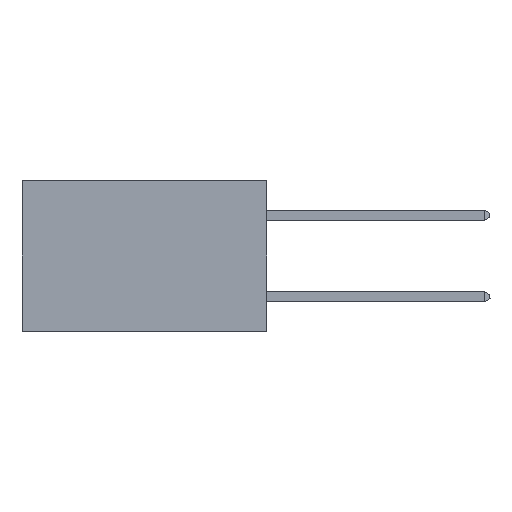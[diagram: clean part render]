
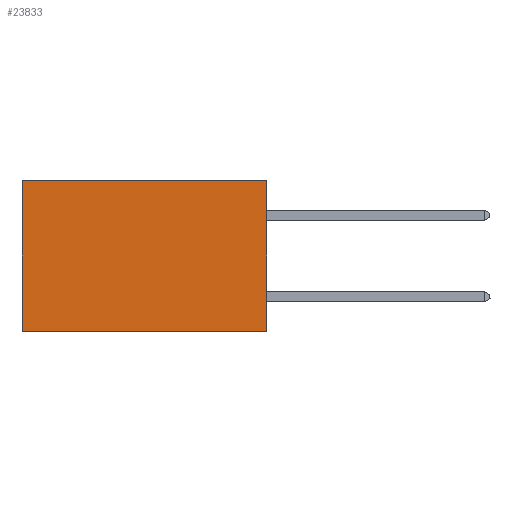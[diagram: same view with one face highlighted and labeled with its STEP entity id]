
A CAD part, left-side view. The second image highlights one B-rep face of the part: STEP entity #23833.
In plain terms, the highlighted planar face has unit normal (-1, 0, 0).
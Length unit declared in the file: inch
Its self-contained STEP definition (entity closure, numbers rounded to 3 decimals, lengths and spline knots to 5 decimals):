
#265 = VERTEX_POINT ( 'NONE', #5550 ) ;
#536 = EDGE_CURVE ( 'NONE', #12801, #21886, #4469, .T. ) ;
#2067 = DIRECTION ( 'NONE',  ( 0., 0., -1. ) ) ;
#2367 = LINE ( 'NONE', #5290, #14525 ) ;
#3176 = CARTESIAN_POINT ( 'NONE',  ( 0.2875, 0., -0.37 ) ) ;
#3340 = ORIENTED_EDGE ( 'NONE', *, *, #536, .T. ) ;
#3787 = LINE ( 'NONE', #24028, #14053 ) ;
#4469 = LINE ( 'NONE', #28018, #17344 ) ;
#5175 = PLANE ( 'NONE',  #5672 ) ;
#5278 = EDGE_LOOP ( 'NONE', ( #3340, #19944, #5792, #25168 ) ) ;
#5290 = CARTESIAN_POINT ( 'NONE',  ( 0.2875, 0., 0. ) ) ;
#5550 = CARTESIAN_POINT ( 'NONE',  ( 0.2875, 0., 0. ) ) ;
#5672 = AXIS2_PLACEMENT_3D ( 'NONE', #27418, #12820, #7746 ) ;
#5792 = ORIENTED_EDGE ( 'NONE', *, *, #21188, .F. ) ;
#7746 = DIRECTION ( 'NONE',  ( 0., 0., -1. ) ) ;
#9611 = DIRECTION ( 'NONE',  ( 0., 1., 0. ) ) ;
#11300 = VERTEX_POINT ( 'NONE', #3176 ) ;
#12801 = VERTEX_POINT ( 'NONE', #23827 ) ;
#12820 = DIRECTION ( 'NONE',  ( 1., 0., 0. ) ) ;
#13310 = LINE ( 'NONE', #20395, #13675 ) ;
#13675 = VECTOR ( 'NONE', #25488, 39.37008 ) ;
#14053 = VECTOR ( 'NONE', #9611, 39.37008 ) ;
#14525 = VECTOR ( 'NONE', #17608, 39.37008 ) ;
#17344 = VECTOR ( 'NONE', #2067, 39.37008 ) ;
#17608 = DIRECTION ( 'NONE',  ( 0., 1., 0. ) ) ;
#18186 = EDGE_CURVE ( 'NONE', #265, #12801, #2367, .T. ) ;
#19648 = EDGE_CURVE ( 'NONE', #11300, #21886, #3787, .T. ) ;
#19944 = ORIENTED_EDGE ( 'NONE', *, *, #19648, .F. ) ;
#20395 = CARTESIAN_POINT ( 'NONE',  ( 0.2875, 0., 0. ) ) ;
#21188 = EDGE_CURVE ( 'NONE', #265, #11300, #13310, .T. ) ;
#21886 = VERTEX_POINT ( 'NONE', #22570 ) ;
#22570 = CARTESIAN_POINT ( 'NONE',  ( 0.2875, 0.6, -0.37 ) ) ;
#23827 = CARTESIAN_POINT ( 'NONE',  ( 0.2875, 0.6, 0. ) ) ;
#23833 = ADVANCED_FACE ( 'NONE', ( #24528 ), #5175, .F. ) ;
#24028 = CARTESIAN_POINT ( 'NONE',  ( 0.2875, 0., -0.37 ) ) ;
#24528 = FACE_OUTER_BOUND ( 'NONE', #5278, .T. ) ;
#25168 = ORIENTED_EDGE ( 'NONE', *, *, #18186, .T. ) ;
#25488 = DIRECTION ( 'NONE',  ( 0., 0., -1. ) ) ;
#27418 = CARTESIAN_POINT ( 'NONE',  ( 0.2875, 0., 0. ) ) ;
#28018 = CARTESIAN_POINT ( 'NONE',  ( 0.2875, 0.6, 0. ) ) ;
